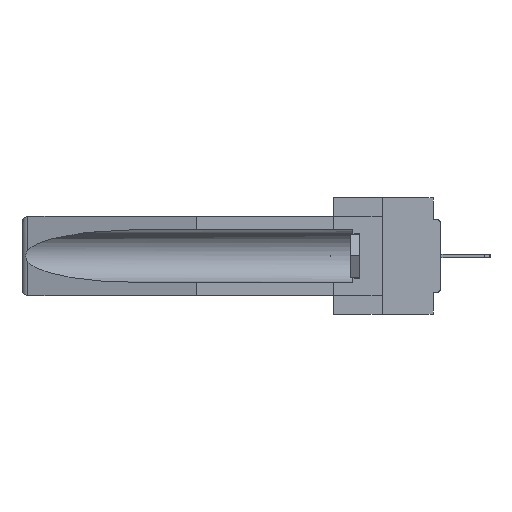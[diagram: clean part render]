
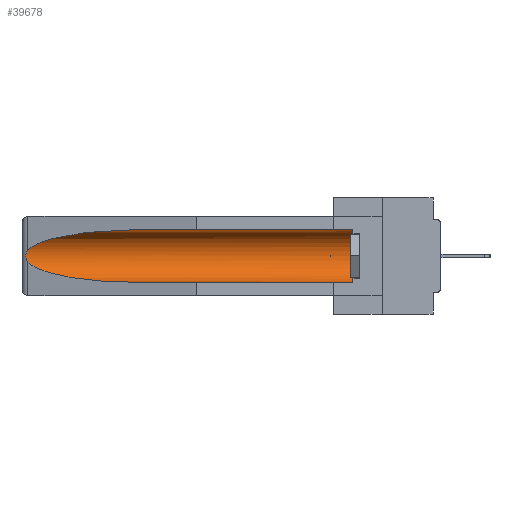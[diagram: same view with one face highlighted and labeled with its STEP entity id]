
A CAD part, left-side view. The second image highlights one B-rep face of the part: STEP entity #39678.
In plain terms, the highlighted cylindrical face has radius 2.857 mm (diameter 5.715 mm), a partial arc.
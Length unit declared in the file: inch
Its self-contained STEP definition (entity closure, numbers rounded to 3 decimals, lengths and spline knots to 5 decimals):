
#999 = ORIENTED_EDGE ( 'NONE', *, *, #19305, .F. ) ;
#2169 = ORIENTED_EDGE ( 'NONE', *, *, #27094, .T. ) ;
#2565 = EDGE_LOOP ( 'NONE', ( #35420, #19903, #29904, #999, #2169, #35494 ) ) ;
#3166 = CARTESIAN_POINT ( 'NONE',  ( 0.21114, 1.30732, -0.059 ) ) ;
#3512 = LINE ( 'NONE', #26021, #25835 ) ;
#4025 = CARTESIAN_POINT ( 'NONE',  ( 0.21114, 1.30732, -0.284 ) ) ;
#5501 = CARTESIAN_POINT ( 'NONE',  ( 0.26537, 1.52718, -0.14972 ) ) ;
#5515 = EDGE_CURVE ( 'NONE', #31529, #14302, #6122, .T. ) ;
#6122 =( BOUNDED_CURVE ( )  B_SPLINE_CURVE ( 3, ( #7607, #13741, #4025, #8011 ),
 .UNSPECIFIED., .F., .T. ) 
 B_SPLINE_CURVE_WITH_KNOTS ( ( 4, 4 ),
 ( 0.1948, 1.5708 ),
 .UNSPECIFIED. ) 
 CURVE ( )  GEOMETRIC_REPRESENTATION_ITEM ( )  RATIONAL_B_SPLINE_CURVE ( ( 1., 0.848, 0.848, 1. ) ) 
 REPRESENTATION_ITEM ( '' )  );
#6185 = AXIS2_PLACEMENT_3D ( 'NONE', #12752, #12972, #8950 ) ;
#6609 = CARTESIAN_POINT ( 'NONE',  ( 0.2675, 1.53308, -0.16763 ) ) ;
#7607 = CARTESIAN_POINT ( 'NONE',  ( 0.26537, 1.52718, -0.19328 ) ) ;
#8011 = CARTESIAN_POINT ( 'NONE',  ( 0.155, 1.07973, -0.284 ) ) ;
#8214 = CIRCLE ( 'NONE', #6185, 0.1125 ) ;
#8950 = DIRECTION ( 'NONE',  ( 0., 0., 1. ) ) ;
#10453 = VERTEX_POINT ( 'NONE', #23580 ) ;
#12752 = CARTESIAN_POINT ( 'NONE',  ( 0.155, 0.126, -0.1715 ) ) ;
#12972 = DIRECTION ( 'NONE',  ( 0., -1., 0. ) ) ;
#13134 = CARTESIAN_POINT ( 'NONE',  ( 0.26537, 1.52718, -0.19328 ) ) ;
#13741 = CARTESIAN_POINT ( 'NONE',  ( 0.25451, 1.48313, -0.24835 ) ) ;
#14302 = VERTEX_POINT ( 'NONE', #38115 ) ;
#15091 = CARTESIAN_POINT ( 'NONE',  ( 0.26597, 1.52961, -0.15275 ) ) ;
#15146 = CARTESIAN_POINT ( 'NONE',  ( 0.155, 0.126, -0.284 ) ) ;
#15792 = B_SPLINE_CURVE_WITH_KNOTS ( 'NONE', 3,
 ( #31065, #15091, #34423, #34823, #6609, #28532, #22023, #16336, #19280, #22226 ),
 .UNSPECIFIED., .F., .F.,
 ( 4, 2, 2, 2, 4 ),
 ( 0., 0.00029, 0.00058, 0.00087, 0.00117 ),
 .UNSPECIFIED. ) ;
#16336 = CARTESIAN_POINT ( 'NONE',  ( 0.26655, 1.53094, -0.18657 ) ) ;
#19280 = CARTESIAN_POINT ( 'NONE',  ( 0.26597, 1.5296, -0.19026 ) ) ;
#19305 = EDGE_CURVE ( 'NONE', #30441, #14302, #3512, .T. ) ;
#19613 = EDGE_CURVE ( 'NONE', #40803, #10453, #39387, .T. ) ;
#19903 = ORIENTED_EDGE ( 'NONE', *, *, #36527, .T. ) ;
#22023 = CARTESIAN_POINT ( 'NONE',  ( 0.2673, 1.53269, -0.17917 ) ) ;
#22226 = CARTESIAN_POINT ( 'NONE',  ( 0.26537, 1.52718, -0.19328 ) ) ;
#23407 = CARTESIAN_POINT ( 'NONE',  ( 0.155, -0.30754, -0.059 ) ) ;
#23580 = CARTESIAN_POINT ( 'NONE',  ( 0.155, 1.07973, -0.059 ) ) ;
#23594 = FACE_OUTER_BOUND ( 'NONE', #2565, .T. ) ;
#24010 = CYLINDRICAL_SURFACE ( 'NONE', #27134, 0.1125 ) ;
#24561 = VERTEX_POINT ( 'NONE', #40243 ) ;
#25835 = VECTOR ( 'NONE', #35926, 39.37008 ) ;
#26021 = CARTESIAN_POINT ( 'NONE',  ( 0.155, -0.30754, -0.284 ) ) ;
#27094 = EDGE_CURVE ( 'NONE', #30441, #40803, #8214, .T. ) ;
#27134 = AXIS2_PLACEMENT_3D ( 'NONE', #27173, #39976, #36418 ) ;
#27173 = CARTESIAN_POINT ( 'NONE',  ( 0.155, -0.30754, -0.1715 ) ) ;
#28532 = CARTESIAN_POINT ( 'NONE',  ( 0.2675, 1.53308, -0.17534 ) ) ;
#29904 = ORIENTED_EDGE ( 'NONE', *, *, #5515, .T. ) ;
#29906 = VECTOR ( 'NONE', #36228, 39.37008 ) ;
#30441 = VERTEX_POINT ( 'NONE', #15146 ) ;
#31065 = CARTESIAN_POINT ( 'NONE',  ( 0.26537, 1.52718, -0.14972 ) ) ;
#31529 = VERTEX_POINT ( 'NONE', #13134 ) ;
#34326 = CARTESIAN_POINT ( 'NONE',  ( 0.25451, 1.48313, -0.09465 ) ) ;
#34423 = CARTESIAN_POINT ( 'NONE',  ( 0.26654, 1.53092, -0.15636 ) ) ;
#34543 = CARTESIAN_POINT ( 'NONE',  ( 0.155, 1.07973, -0.059 ) ) ;
#34823 = CARTESIAN_POINT ( 'NONE',  ( 0.2673, 1.5327, -0.16383 ) ) ;
#35035 = EDGE_CURVE ( 'NONE', #10453, #24561, #37585, .T. ) ;
#35420 = ORIENTED_EDGE ( 'NONE', *, *, #35035, .T. ) ;
#35442 = CARTESIAN_POINT ( 'NONE',  ( 0.155, 0.126, -0.059 ) ) ;
#35494 = ORIENTED_EDGE ( 'NONE', *, *, #19613, .T. ) ;
#35926 = DIRECTION ( 'NONE',  ( 0., 1., 0. ) ) ;
#36228 = DIRECTION ( 'NONE',  ( 0., 1., 0. ) ) ;
#36418 = DIRECTION ( 'NONE',  ( 0., 0., 1. ) ) ;
#36527 = EDGE_CURVE ( 'NONE', #24561, #31529, #15792, .T. ) ;
#37585 =( BOUNDED_CURVE ( )  B_SPLINE_CURVE ( 3, ( #34543, #3166, #34326, #5501 ),
 .UNSPECIFIED., .F., .T. ) 
 B_SPLINE_CURVE_WITH_KNOTS ( ( 4, 4 ),
 ( 4.71239, 6.08839 ),
 .UNSPECIFIED. ) 
 CURVE ( )  GEOMETRIC_REPRESENTATION_ITEM ( )  RATIONAL_B_SPLINE_CURVE ( ( 1., 0.848, 0.848, 1. ) ) 
 REPRESENTATION_ITEM ( '' )  );
#38115 = CARTESIAN_POINT ( 'NONE',  ( 0.155, 1.07973, -0.284 ) ) ;
#39387 = LINE ( 'NONE', #23407, #29906 ) ;
#39678 = ADVANCED_FACE ( 'NONE', ( #23594 ), #24010, .F. ) ;
#39976 = DIRECTION ( 'NONE',  ( 0., 1., 0. ) ) ;
#40243 = CARTESIAN_POINT ( 'NONE',  ( 0.26537, 1.52718, -0.14972 ) ) ;
#40803 = VERTEX_POINT ( 'NONE', #35442 ) ;
